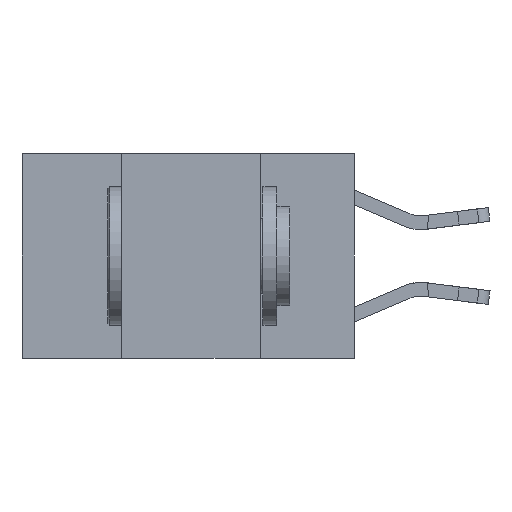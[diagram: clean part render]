
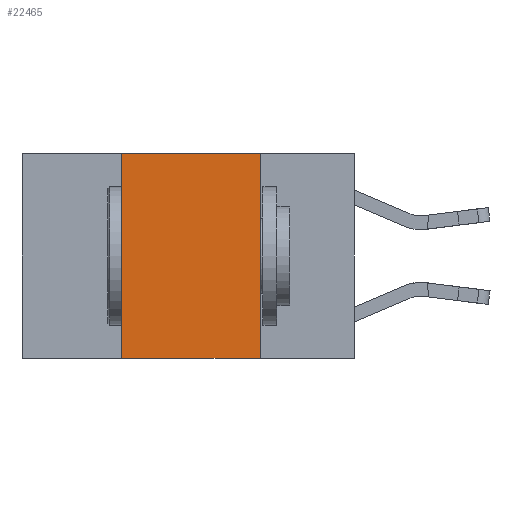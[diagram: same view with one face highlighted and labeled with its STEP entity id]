
A CAD part, left-side view. The second image highlights one B-rep face of the part: STEP entity #22465.
In plain terms, the highlighted planar face has unit normal (-1, 0, 0).
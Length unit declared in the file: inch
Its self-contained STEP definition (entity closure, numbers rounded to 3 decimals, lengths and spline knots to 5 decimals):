
#1041 = EDGE_CURVE ( 'NONE', #8105, #10286, #4743, .T. ) ;
#1464 = CARTESIAN_POINT ( 'NONE',  ( 0., 0.17, 0. ) ) ;
#3166 = DIRECTION ( 'NONE',  ( 0., -1., 0. ) ) ;
#3933 = DIRECTION ( 'NONE',  ( 0., -1., 0. ) ) ;
#4445 = VECTOR ( 'NONE', #3166, 39.37008 ) ;
#4743 = LINE ( 'NONE', #6489, #27449 ) ;
#4882 = LINE ( 'NONE', #8390, #16648 ) ;
#6282 = ORIENTED_EDGE ( 'NONE', *, *, #12558, .F. ) ;
#6489 = CARTESIAN_POINT ( 'NONE',  ( 0., 0.42, 0. ) ) ;
#7559 = EDGE_CURVE ( 'NONE', #8105, #12403, #16171, .T. ) ;
#7818 = FACE_OUTER_BOUND ( 'NONE', #25050, .T. ) ;
#8105 = VERTEX_POINT ( 'NONE', #25124 ) ;
#8390 = CARTESIAN_POINT ( 'NONE',  ( 0., 0.6, 0. ) ) ;
#9670 = DIRECTION ( 'NONE',  ( 0., 0., 1. ) ) ;
#9944 = DIRECTION ( 'NONE',  ( 0., 0., -1. ) ) ;
#10286 = VERTEX_POINT ( 'NONE', #21650 ) ;
#12141 = ORIENTED_EDGE ( 'NONE', *, *, #27614, .F. ) ;
#12403 = VERTEX_POINT ( 'NONE', #27905 ) ;
#12558 = EDGE_CURVE ( 'NONE', #23345, #12403, #22409, .T. ) ;
#15453 = DIRECTION ( 'NONE',  ( 0., 0., -1. ) ) ;
#16171 = LINE ( 'NONE', #16406, #4445 ) ;
#16406 = CARTESIAN_POINT ( 'NONE',  ( 0., 0.6, -0.37 ) ) ;
#16529 = CARTESIAN_POINT ( 'NONE',  ( 0., 0.6, 0. ) ) ;
#16540 = VECTOR ( 'NONE', #15453, 39.37008 ) ;
#16648 = VECTOR ( 'NONE', #3933, 39.37008 ) ;
#20877 = PLANE ( 'NONE',  #25273 ) ;
#21650 = CARTESIAN_POINT ( 'NONE',  ( 0., 0.42, 0. ) ) ;
#22409 = LINE ( 'NONE', #24153, #16540 ) ;
#22465 = ADVANCED_FACE ( 'NONE', ( #7818 ), #20877, .F. ) ;
#23171 = DIRECTION ( 'NONE',  ( 1., 0., 0. ) ) ;
#23345 = VERTEX_POINT ( 'NONE', #1464 ) ;
#23847 = ORIENTED_EDGE ( 'NONE', *, *, #7559, .T. ) ;
#24153 = CARTESIAN_POINT ( 'NONE',  ( 0., 0.17, 0. ) ) ;
#24179 = ORIENTED_EDGE ( 'NONE', *, *, #1041, .F. ) ;
#25050 = EDGE_LOOP ( 'NONE', ( #6282, #12141, #24179, #23847 ) ) ;
#25124 = CARTESIAN_POINT ( 'NONE',  ( 0., 0.42, -0.37 ) ) ;
#25273 = AXIS2_PLACEMENT_3D ( 'NONE', #16529, #23171, #9944 ) ;
#27449 = VECTOR ( 'NONE', #9670, 39.37008 ) ;
#27614 = EDGE_CURVE ( 'NONE', #10286, #23345, #4882, .T. ) ;
#27905 = CARTESIAN_POINT ( 'NONE',  ( 0., 0.17, -0.37 ) ) ;
